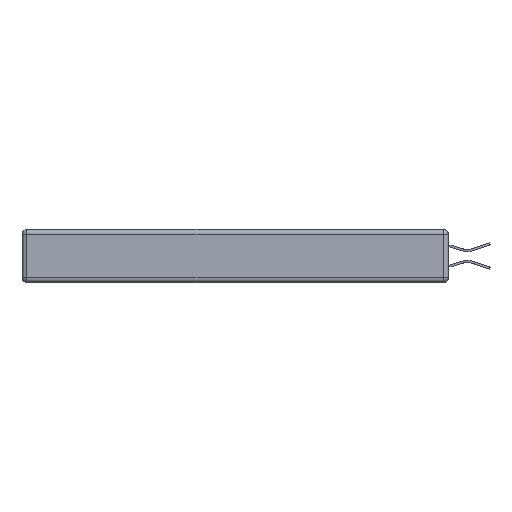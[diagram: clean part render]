
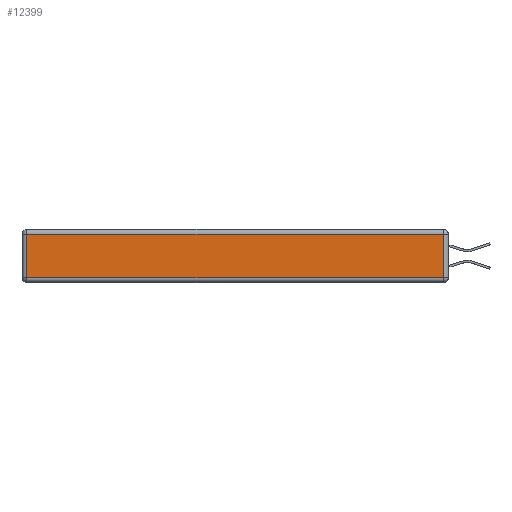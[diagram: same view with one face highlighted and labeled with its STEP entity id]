
A CAD part, left-side view. The second image highlights one B-rep face of the part: STEP entity #12399.
In plain terms, the highlighted planar face has unit normal (-1, 0, 0).
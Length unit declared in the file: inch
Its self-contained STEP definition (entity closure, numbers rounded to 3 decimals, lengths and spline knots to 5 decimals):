
#564 = ORIENTED_EDGE ( 'NONE', *, *, #18285, .T. ) ;
#1486 = FACE_OUTER_BOUND ( 'NONE', #6879, .T. ) ;
#1939 = DIRECTION ( 'NONE',  ( 0., -1., 0. ) ) ;
#2334 = CARTESIAN_POINT ( 'NONE',  ( 0., 0.03, -0.313 ) ) ;
#3113 = DIRECTION ( 'NONE',  ( 0., 0., -1. ) ) ;
#3440 = EDGE_CURVE ( 'NONE', #9458, #12141, #4059, .T. ) ;
#4059 = LINE ( 'NONE', #4629, #20033 ) ;
#4629 = CARTESIAN_POINT ( 'NONE',  ( 0., 2.72, -0.343 ) ) ;
#5124 = CARTESIAN_POINT ( 'NONE',  ( 0., 0.03, -0.343 ) ) ;
#5149 = ORIENTED_EDGE ( 'NONE', *, *, #18264, .T. ) ;
#5698 = LINE ( 'NONE', #8080, #6648 ) ;
#6266 = CARTESIAN_POINT ( 'NONE',  ( 0., 2.75, -0.03 ) ) ;
#6648 = VECTOR ( 'NONE', #1939, 39.37008 ) ;
#6879 = EDGE_LOOP ( 'NONE', ( #564, #14869, #5149, #13750 ) ) ;
#8080 = CARTESIAN_POINT ( 'NONE',  ( 0., 0., -0.313 ) ) ;
#8332 = VECTOR ( 'NONE', #9373, 39.37008 ) ;
#8839 = LINE ( 'NONE', #6266, #8332 ) ;
#9373 = DIRECTION ( 'NONE',  ( 0., 1., 0. ) ) ;
#9458 = VERTEX_POINT ( 'NONE', #14415 ) ;
#10176 = DIRECTION ( 'NONE',  ( -1., 0., 0. ) ) ;
#10802 = VERTEX_POINT ( 'NONE', #2334 ) ;
#10936 = VERTEX_POINT ( 'NONE', #14474 ) ;
#12141 = VERTEX_POINT ( 'NONE', #14089 ) ;
#12358 = AXIS2_PLACEMENT_3D ( 'NONE', #17862, #10176, #13054 ) ;
#12399 = ADVANCED_FACE ( 'NONE', ( #1486 ), #17926, .T. ) ;
#13054 = DIRECTION ( 'NONE',  ( 0., 0., 1. ) ) ;
#13750 = ORIENTED_EDGE ( 'NONE', *, *, #3440, .T. ) ;
#13971 = VECTOR ( 'NONE', #14490, 39.37008 ) ;
#14089 = CARTESIAN_POINT ( 'NONE',  ( 0., 2.72, -0.313 ) ) ;
#14415 = CARTESIAN_POINT ( 'NONE',  ( 0., 2.72, -0.03 ) ) ;
#14474 = CARTESIAN_POINT ( 'NONE',  ( 0., 0.03, -0.03 ) ) ;
#14490 = DIRECTION ( 'NONE',  ( 0., 0., 1. ) ) ;
#14869 = ORIENTED_EDGE ( 'NONE', *, *, #17014, .T. ) ;
#17014 = EDGE_CURVE ( 'NONE', #10802, #10936, #19522, .T. ) ;
#17862 = CARTESIAN_POINT ( 'NONE',  ( 0., 0., -0.343 ) ) ;
#17926 = PLANE ( 'NONE',  #12358 ) ;
#18264 = EDGE_CURVE ( 'NONE', #10936, #9458, #8839, .T. ) ;
#18285 = EDGE_CURVE ( 'NONE', #12141, #10802, #5698, .T. ) ;
#19522 = LINE ( 'NONE', #5124, #13971 ) ;
#20033 = VECTOR ( 'NONE', #3113, 39.37008 ) ;
